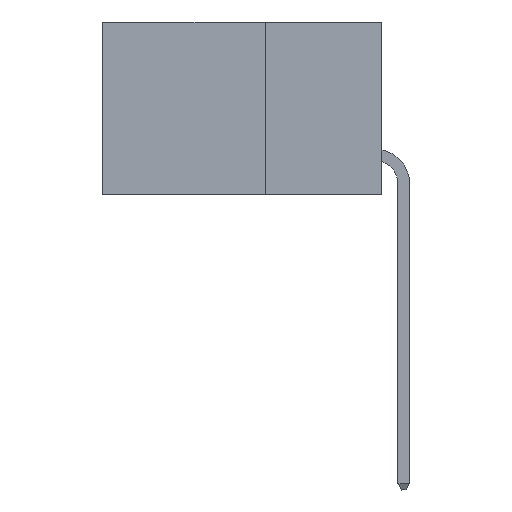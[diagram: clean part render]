
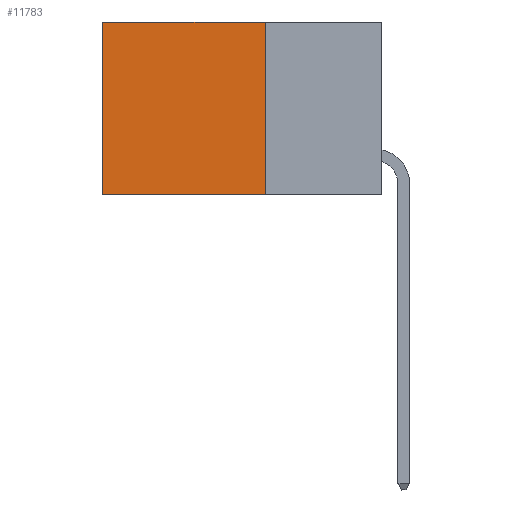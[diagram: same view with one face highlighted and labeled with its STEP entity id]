
A CAD part, left-side view. The second image highlights one B-rep face of the part: STEP entity #11783.
In plain terms, the highlighted planar face has unit normal (-1, 0, 0).
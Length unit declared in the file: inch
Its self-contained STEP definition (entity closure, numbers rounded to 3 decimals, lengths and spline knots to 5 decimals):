
#96 = DIRECTION ( 'NONE',  ( 0., 0., -1. ) ) ;
#1623 = VECTOR ( 'NONE', #7735, 39.37008 ) ;
#2389 = CARTESIAN_POINT ( 'NONE',  ( 0.2875, 0.25, 0. ) ) ;
#2777 = VERTEX_POINT ( 'NONE', #2389 ) ;
#2796 = CARTESIAN_POINT ( 'NONE',  ( 0.2875, 0.6, 0. ) ) ;
#4148 = VECTOR ( 'NONE', #96, 39.37008 ) ;
#4582 = EDGE_CURVE ( 'NONE', #2777, #9022, #8897, .T. ) ;
#5804 = ORIENTED_EDGE ( 'NONE', *, *, #4582, .F. ) ;
#5904 = AXIS2_PLACEMENT_3D ( 'NONE', #16631, #17980, #7768 ) ;
#6277 = CARTESIAN_POINT ( 'NONE',  ( 0.2875, 0.25, 0. ) ) ;
#6761 = EDGE_CURVE ( 'NONE', #8241, #12145, #7398, .T. ) ;
#7398 = LINE ( 'NONE', #12167, #4148 ) ;
#7735 = DIRECTION ( 'NONE',  ( 0., 1., 0. ) ) ;
#7768 = DIRECTION ( 'NONE',  ( 0., 0., -1. ) ) ;
#8241 = VERTEX_POINT ( 'NONE', #2796 ) ;
#8803 = ORIENTED_EDGE ( 'NONE', *, *, #12953, .T. ) ;
#8814 = LINE ( 'NONE', #6277, #11183 ) ;
#8897 = LINE ( 'NONE', #9982, #18462 ) ;
#9022 = VERTEX_POINT ( 'NONE', #17999 ) ;
#9029 = ORIENTED_EDGE ( 'NONE', *, *, #18307, .F. ) ;
#9982 = CARTESIAN_POINT ( 'NONE',  ( 0.2875, 0.25, 0. ) ) ;
#11183 = VECTOR ( 'NONE', #18335, 39.37008 ) ;
#11216 = ORIENTED_EDGE ( 'NONE', *, *, #6761, .T. ) ;
#11221 = EDGE_LOOP ( 'NONE', ( #11216, #9029, #5804, #8803 ) ) ;
#11294 = DIRECTION ( 'NONE',  ( 0., 0., -1. ) ) ;
#11720 = CARTESIAN_POINT ( 'NONE',  ( 0.2875, 0.6, -0.37 ) ) ;
#11783 = ADVANCED_FACE ( 'NONE', ( #11912 ), #12214, .F. ) ;
#11912 = FACE_OUTER_BOUND ( 'NONE', #11221, .T. ) ;
#12145 = VERTEX_POINT ( 'NONE', #11720 ) ;
#12167 = CARTESIAN_POINT ( 'NONE',  ( 0.2875, 0.6, 0. ) ) ;
#12214 = PLANE ( 'NONE',  #5904 ) ;
#12953 = EDGE_CURVE ( 'NONE', #2777, #8241, #8814, .T. ) ;
#15122 = LINE ( 'NONE', #15169, #1623 ) ;
#15169 = CARTESIAN_POINT ( 'NONE',  ( 0.2875, 0.25, -0.37 ) ) ;
#16631 = CARTESIAN_POINT ( 'NONE',  ( 0.2875, 0.25, 0. ) ) ;
#17980 = DIRECTION ( 'NONE',  ( 1., 0., 0. ) ) ;
#17999 = CARTESIAN_POINT ( 'NONE',  ( 0.2875, 0.25, -0.37 ) ) ;
#18307 = EDGE_CURVE ( 'NONE', #9022, #12145, #15122, .T. ) ;
#18335 = DIRECTION ( 'NONE',  ( 0., 1., 0. ) ) ;
#18462 = VECTOR ( 'NONE', #11294, 39.37008 ) ;
